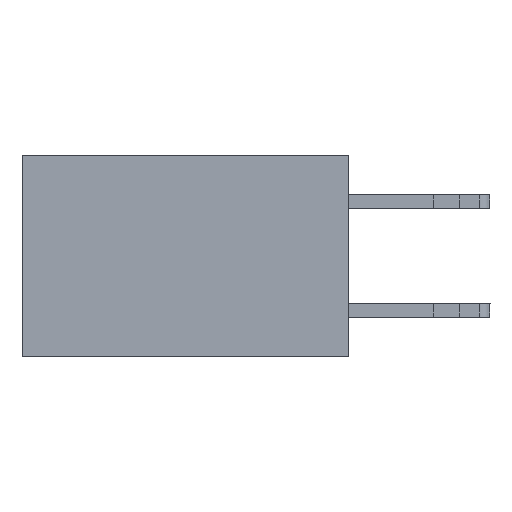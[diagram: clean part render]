
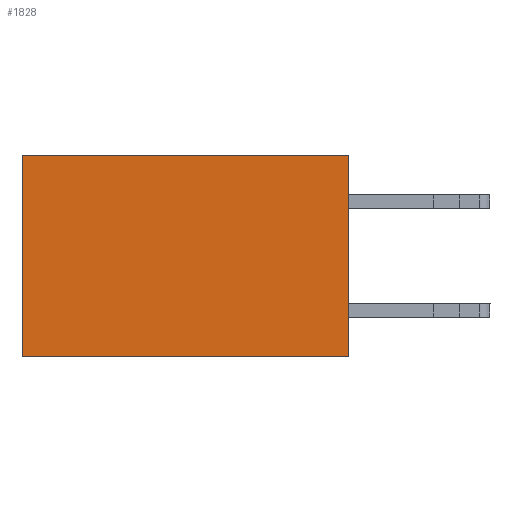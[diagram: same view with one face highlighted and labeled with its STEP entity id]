
A CAD part, left-side view. The second image highlights one B-rep face of the part: STEP entity #1828.
In plain terms, the highlighted planar face has unit normal (-1, 0, 0).
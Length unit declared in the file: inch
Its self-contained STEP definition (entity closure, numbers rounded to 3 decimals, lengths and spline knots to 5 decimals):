
#1582 = CARTESIAN_POINT ( 'NONE',  ( 0.2615, 0., -0.37 ) ) ;
#1584 = ORIENTED_EDGE ( 'NONE', *, *, #5698, .T. ) ;
#1828 = ADVANCED_FACE ( 'NONE', ( #2971 ), #4229, .F. ) ;
#1991 = CARTESIAN_POINT ( 'NONE',  ( 0.2615, 0.6, -0.37 ) ) ;
#2448 = VECTOR ( 'NONE', #10635, 39.37008 ) ;
#2971 = FACE_OUTER_BOUND ( 'NONE', #14157, .T. ) ;
#4196 = VECTOR ( 'NONE', #5175, 39.37008 ) ;
#4229 = PLANE ( 'NONE',  #9332 ) ;
#4500 = EDGE_CURVE ( 'NONE', #5277, #13518, #8579, .T. ) ;
#4801 = VERTEX_POINT ( 'NONE', #9265 ) ;
#4864 = ORIENTED_EDGE ( 'NONE', *, *, #5722, .F. ) ;
#5022 = DIRECTION ( 'NONE',  ( 0., 0., -1. ) ) ;
#5041 = DIRECTION ( 'NONE',  ( 1., 0., 0. ) ) ;
#5061 = DIRECTION ( 'NONE',  ( 0., 1., 0. ) ) ;
#5071 = CARTESIAN_POINT ( 'NONE',  ( 0.2615, 0., -0.37 ) ) ;
#5160 = CARTESIAN_POINT ( 'NONE',  ( 0.2615, 0.6, -0.37 ) ) ;
#5175 = DIRECTION ( 'NONE',  ( 0., 0., -1. ) ) ;
#5277 = VERTEX_POINT ( 'NONE', #7338 ) ;
#5330 = VECTOR ( 'NONE', #8141, 39.37008 ) ;
#5698 = EDGE_CURVE ( 'NONE', #4801, #6350, #10057, .T. ) ;
#5722 = EDGE_CURVE ( 'NONE', #13518, #6350, #10380, .T. ) ;
#6350 = VERTEX_POINT ( 'NONE', #1991 ) ;
#7338 = CARTESIAN_POINT ( 'NONE',  ( 0.2615, 0., 0. ) ) ;
#8141 = DIRECTION ( 'NONE',  ( 0., 1., 0. ) ) ;
#8579 = LINE ( 'NONE', #10606, #2448 ) ;
#9265 = CARTESIAN_POINT ( 'NONE',  ( 0.2615, 0.6, 0. ) ) ;
#9332 = AXIS2_PLACEMENT_3D ( 'NONE', #1582, #5041, #5022 ) ;
#9507 = CARTESIAN_POINT ( 'NONE',  ( 0.2615, 0., 0. ) ) ;
#10057 = LINE ( 'NONE', #5160, #4196 ) ;
#10373 = EDGE_CURVE ( 'NONE', #5277, #4801, #11095, .T. ) ;
#10380 = LINE ( 'NONE', #5071, #12799 ) ;
#10501 = CARTESIAN_POINT ( 'NONE',  ( 0.2615, 0., -0.37 ) ) ;
#10606 = CARTESIAN_POINT ( 'NONE',  ( 0.2615, 0., -0.37 ) ) ;
#10635 = DIRECTION ( 'NONE',  ( 0., 0., -1. ) ) ;
#10681 = ORIENTED_EDGE ( 'NONE', *, *, #4500, .F. ) ;
#11095 = LINE ( 'NONE', #9507, #5330 ) ;
#12799 = VECTOR ( 'NONE', #5061, 39.37008 ) ;
#13389 = ORIENTED_EDGE ( 'NONE', *, *, #10373, .T. ) ;
#13518 = VERTEX_POINT ( 'NONE', #10501 ) ;
#14157 = EDGE_LOOP ( 'NONE', ( #1584, #4864, #10681, #13389 ) ) ;
